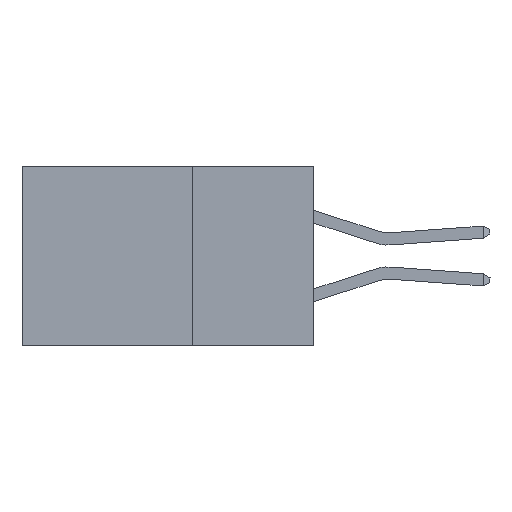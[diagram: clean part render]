
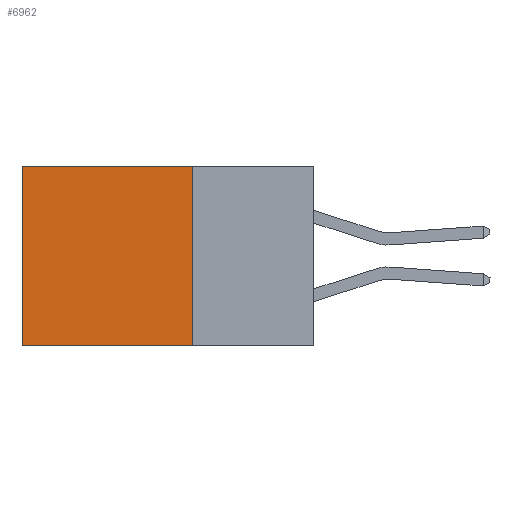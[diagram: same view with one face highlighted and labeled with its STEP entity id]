
A CAD part, left-side view. The second image highlights one B-rep face of the part: STEP entity #6962.
In plain terms, the highlighted planar face has unit normal (-1, 0, 0).
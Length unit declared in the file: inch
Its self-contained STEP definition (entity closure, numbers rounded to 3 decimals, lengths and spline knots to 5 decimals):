
#719 = DIRECTION ( 'NONE',  ( 0., 0., -1. ) ) ;
#1195 = DIRECTION ( 'NONE',  ( 1., 0., 0. ) ) ;
#1340 = LINE ( 'NONE', #6386, #8209 ) ;
#1760 = VERTEX_POINT ( 'NONE', #3998 ) ;
#2326 = ORIENTED_EDGE ( 'NONE', *, *, #6219, .F. ) ;
#2861 = CARTESIAN_POINT ( 'NONE',  ( 0.2875, 0.6, 0. ) ) ;
#3002 = VECTOR ( 'NONE', #10267, 39.37008 ) ;
#3212 = CARTESIAN_POINT ( 'NONE',  ( 0.2875, 0.6, 0. ) ) ;
#3235 = FACE_OUTER_BOUND ( 'NONE', #3328, .T. ) ;
#3255 = LINE ( 'NONE', #9456, #3002 ) ;
#3328 = EDGE_LOOP ( 'NONE', ( #6388, #8955, #2326, #4611 ) ) ;
#3670 = EDGE_CURVE ( 'NONE', #3952, #7890, #1340, .T. ) ;
#3952 = VERTEX_POINT ( 'NONE', #6251 ) ;
#3998 = CARTESIAN_POINT ( 'NONE',  ( 0.2875, 0.25, 0. ) ) ;
#4611 = ORIENTED_EDGE ( 'NONE', *, *, #7662, .T. ) ;
#5136 = CARTESIAN_POINT ( 'NONE',  ( 0.2875, 0.25, 0. ) ) ;
#5423 = CARTESIAN_POINT ( 'NONE',  ( 0.2875, 0.25, 0. ) ) ;
#5648 = VECTOR ( 'NONE', #719, 39.37008 ) ;
#5796 = VERTEX_POINT ( 'NONE', #2861 ) ;
#6127 = AXIS2_PLACEMENT_3D ( 'NONE', #5423, #1195, #7206 ) ;
#6219 = EDGE_CURVE ( 'NONE', #1760, #3952, #3255, .T. ) ;
#6251 = CARTESIAN_POINT ( 'NONE',  ( 0.2875, 0.25, -0.37 ) ) ;
#6386 = CARTESIAN_POINT ( 'NONE',  ( 0.2875, 0.25, -0.37 ) ) ;
#6388 = ORIENTED_EDGE ( 'NONE', *, *, #7159, .T. ) ;
#6544 = CARTESIAN_POINT ( 'NONE',  ( 0.2875, 0.6, -0.37 ) ) ;
#6962 = ADVANCED_FACE ( 'NONE', ( #3235 ), #10533, .F. ) ;
#7159 = EDGE_CURVE ( 'NONE', #5796, #7890, #8257, .T. ) ;
#7206 = DIRECTION ( 'NONE',  ( 0., 0., -1. ) ) ;
#7662 = EDGE_CURVE ( 'NONE', #1760, #5796, #8260, .T. ) ;
#7890 = VERTEX_POINT ( 'NONE', #6544 ) ;
#8209 = VECTOR ( 'NONE', #9491, 39.37008 ) ;
#8257 = LINE ( 'NONE', #3212, #5648 ) ;
#8260 = LINE ( 'NONE', #5136, #10199 ) ;
#8955 = ORIENTED_EDGE ( 'NONE', *, *, #3670, .F. ) ;
#9456 = CARTESIAN_POINT ( 'NONE',  ( 0.2875, 0.25, 0. ) ) ;
#9491 = DIRECTION ( 'NONE',  ( 0., 1., 0. ) ) ;
#10199 = VECTOR ( 'NONE', #10265, 39.37008 ) ;
#10265 = DIRECTION ( 'NONE',  ( 0., 1., 0. ) ) ;
#10267 = DIRECTION ( 'NONE',  ( 0., 0., -1. ) ) ;
#10533 = PLANE ( 'NONE',  #6127 ) ;
